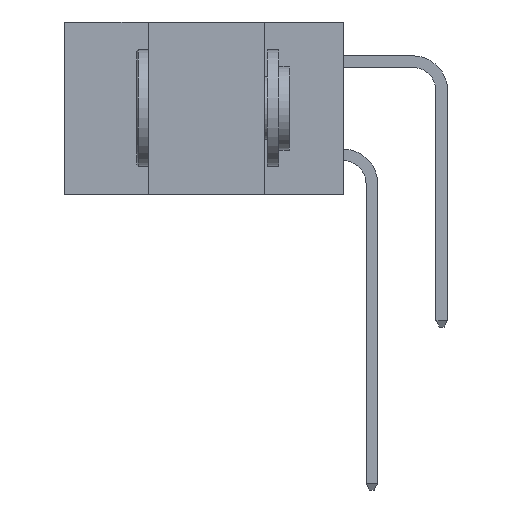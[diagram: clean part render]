
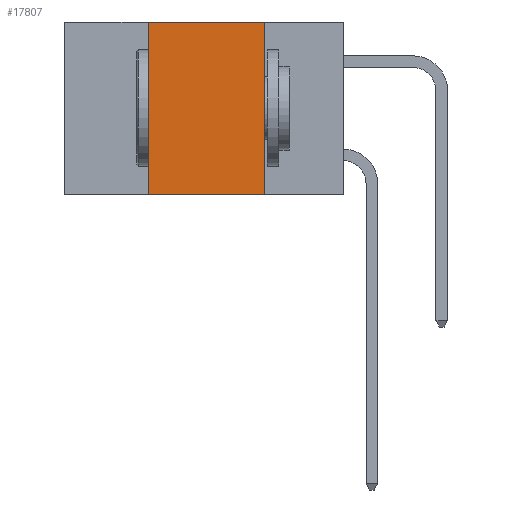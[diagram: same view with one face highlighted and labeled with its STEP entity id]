
A CAD part, left-side view. The second image highlights one B-rep face of the part: STEP entity #17807.
In plain terms, the highlighted planar face has unit normal (-1, 0, 0).
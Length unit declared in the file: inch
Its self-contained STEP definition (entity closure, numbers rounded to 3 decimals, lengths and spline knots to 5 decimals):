
#2141 = EDGE_CURVE ( 'NONE', #26688, #5937, #26577, .T. ) ;
#2989 = ORIENTED_EDGE ( 'NONE', *, *, #2141, .F. ) ;
#3397 = CARTESIAN_POINT ( 'NONE',  ( 0., 0.17, 0. ) ) ;
#4302 = DIRECTION ( 'NONE',  ( 0., -1., 0. ) ) ;
#4343 = LINE ( 'NONE', #8014, #24586 ) ;
#5937 = VERTEX_POINT ( 'NONE', #21176 ) ;
#6986 = VECTOR ( 'NONE', #4302, 39.37008 ) ;
#8014 = CARTESIAN_POINT ( 'NONE',  ( 0., 0.17, -0.37 ) ) ;
#8317 = CARTESIAN_POINT ( 'NONE',  ( 0., 0.6, -0.37 ) ) ;
#8639 = ORIENTED_EDGE ( 'NONE', *, *, #24113, .T. ) ;
#9044 = VERTEX_POINT ( 'NONE', #3397 ) ;
#10170 = EDGE_LOOP ( 'NONE', ( #24278, #19453, #2989, #8639 ) ) ;
#11118 = DIRECTION ( 'NONE',  ( 1., 0., 0. ) ) ;
#11647 = AXIS2_PLACEMENT_3D ( 'NONE', #19647, #11118, #25825 ) ;
#13261 = FACE_OUTER_BOUND ( 'NONE', #10170, .T. ) ;
#13779 = EDGE_CURVE ( 'NONE', #5937, #9044, #22087, .T. ) ;
#14849 = VECTOR ( 'NONE', #20428, 39.37008 ) ;
#15367 = VERTEX_POINT ( 'NONE', #19753 ) ;
#17807 = ADVANCED_FACE ( 'NONE', ( #13261 ), #23772, .F. ) ;
#18509 = LINE ( 'NONE', #8317, #19166 ) ;
#19166 = VECTOR ( 'NONE', #21193, 39.37008 ) ;
#19353 = CARTESIAN_POINT ( 'NONE',  ( 0., 0.6, 0. ) ) ;
#19453 = ORIENTED_EDGE ( 'NONE', *, *, #13779, .F. ) ;
#19456 = EDGE_CURVE ( 'NONE', #9044, #15367, #4343, .T. ) ;
#19647 = CARTESIAN_POINT ( 'NONE',  ( 0., 0.6, 0. ) ) ;
#19753 = CARTESIAN_POINT ( 'NONE',  ( 0., 0.17, -0.37 ) ) ;
#20428 = DIRECTION ( 'NONE',  ( 0., 0., 1. ) ) ;
#20854 = CARTESIAN_POINT ( 'NONE',  ( 0., 0.42, -0.37 ) ) ;
#21176 = CARTESIAN_POINT ( 'NONE',  ( 0., 0.42, 0. ) ) ;
#21193 = DIRECTION ( 'NONE',  ( 0., -1., 0. ) ) ;
#21752 = CARTESIAN_POINT ( 'NONE',  ( 0., 0.42, -0.37 ) ) ;
#22087 = LINE ( 'NONE', #19353, #6986 ) ;
#23772 = PLANE ( 'NONE',  #11647 ) ;
#24113 = EDGE_CURVE ( 'NONE', #26688, #15367, #18509, .T. ) ;
#24278 = ORIENTED_EDGE ( 'NONE', *, *, #19456, .F. ) ;
#24586 = VECTOR ( 'NONE', #27103, 39.37008 ) ;
#25825 = DIRECTION ( 'NONE',  ( 0., 0., -1. ) ) ;
#26577 = LINE ( 'NONE', #20854, #14849 ) ;
#26688 = VERTEX_POINT ( 'NONE', #21752 ) ;
#27103 = DIRECTION ( 'NONE',  ( 0., 0., -1. ) ) ;
